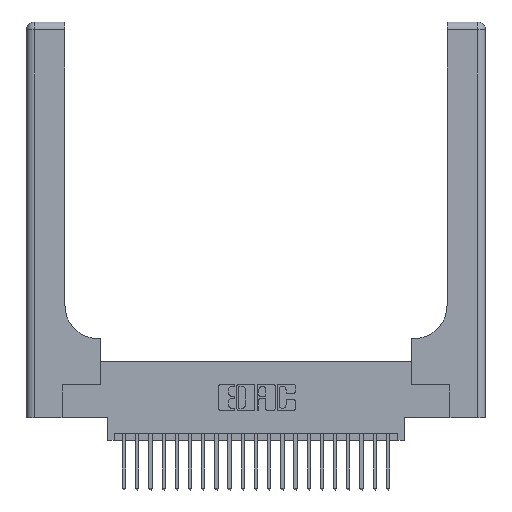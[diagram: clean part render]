
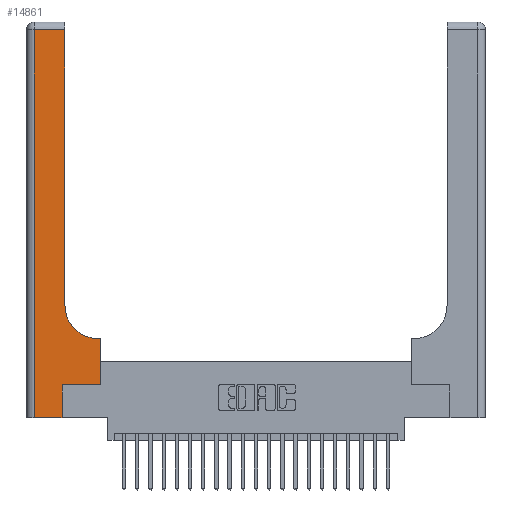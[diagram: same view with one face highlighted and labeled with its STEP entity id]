
A CAD part, top view. The second image highlights one B-rep face of the part: STEP entity #14861.
In plain terms, the highlighted planar face has unit normal (0, 0, 1).
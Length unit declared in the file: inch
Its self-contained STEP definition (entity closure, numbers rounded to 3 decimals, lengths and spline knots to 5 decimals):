
#70 = EDGE_LOOP ( 'NONE', ( #8513, #16734, #17218, #14912, #22025, #20427, #16551, #17496, #13132 ) ) ;
#830 = DIRECTION ( 'NONE',  ( -1., 0., 0. ) ) ;
#1219 = VECTOR ( 'NONE', #1689, 39.37008 ) ;
#1689 = DIRECTION ( 'NONE',  ( 1., 0., 0. ) ) ;
#1909 = VERTEX_POINT ( 'NONE', #11282 ) ;
#2113 = VERTEX_POINT ( 'NONE', #3494 ) ;
#2597 = VERTEX_POINT ( 'NONE', #21710 ) ;
#2657 = DIRECTION ( 'NONE',  ( 0., 0., -1. ) ) ;
#2665 = EDGE_CURVE ( 'NONE', #18563, #23103, #17933, .T. ) ;
#2709 = CARTESIAN_POINT ( 'NONE',  ( 0.5585, 0.25, 0.37 ) ) ;
#2771 = VECTOR ( 'NONE', #12998, 39.37008 ) ;
#3073 = FACE_OUTER_BOUND ( 'NONE', #70, .T. ) ;
#3276 = CIRCLE ( 'NONE', #20025, 0.25 ) ;
#3494 = CARTESIAN_POINT ( 'NONE',  ( 0.06, 2.94, 0.37 ) ) ;
#3606 = AXIS2_PLACEMENT_3D ( 'NONE', #9841, #6160, #8169 ) ;
#4570 = DIRECTION ( 'NONE',  ( 0., 1., 0. ) ) ;
#4891 = VECTOR ( 'NONE', #8653, 39.37008 ) ;
#5004 = EDGE_CURVE ( 'NONE', #17269, #2597, #8825, .T. ) ;
#5356 = VECTOR ( 'NONE', #14593, 39.37008 ) ;
#5906 = CARTESIAN_POINT ( 'NONE',  ( 0.06, 0., 0.37 ) ) ;
#6115 = EDGE_CURVE ( 'NONE', #1909, #17347, #9120, .T. ) ;
#6160 = DIRECTION ( 'NONE',  ( 0., 0., -1. ) ) ;
#6515 = LINE ( 'NONE', #20076, #21144 ) ;
#7162 = CARTESIAN_POINT ( 'NONE',  ( 0.2915, 3., 0.37 ) ) ;
#8169 = DIRECTION ( 'NONE',  ( -1., 0., 0. ) ) ;
#8288 = CARTESIAN_POINT ( 'NONE',  ( 0.5415, 0.85, 0.37 ) ) ;
#8387 = EDGE_CURVE ( 'NONE', #24023, #1909, #12891, .T. ) ;
#8513 = ORIENTED_EDGE ( 'NONE', *, *, #2665, .T. ) ;
#8653 = DIRECTION ( 'NONE',  ( 1., 0., 0. ) ) ;
#8825 = LINE ( 'NONE', #21282, #21071 ) ;
#9120 = LINE ( 'NONE', #22345, #4891 ) ;
#9154 = CARTESIAN_POINT ( 'NONE',  ( 0.269, 0., 0.37 ) ) ;
#9619 = EDGE_CURVE ( 'NONE', #2597, #18563, #3276, .T. ) ;
#9841 = CARTESIAN_POINT ( 'NONE',  ( 0., 3., 0.37 ) ) ;
#10125 = DIRECTION ( 'NONE',  ( 0., -1., 0. ) ) ;
#10188 = EDGE_CURVE ( 'NONE', #12968, #24023, #21439, .T. ) ;
#10872 = LINE ( 'NONE', #17648, #18021 ) ;
#10976 = CARTESIAN_POINT ( 'NONE',  ( 0.269, 0., 0.37 ) ) ;
#11282 = CARTESIAN_POINT ( 'NONE',  ( 0.269, 0.25, 0.37 ) ) ;
#11956 = LINE ( 'NONE', #2709, #17920 ) ;
#12891 = LINE ( 'NONE', #9154, #2771 ) ;
#12968 = VERTEX_POINT ( 'NONE', #5906 ) ;
#12998 = DIRECTION ( 'NONE',  ( 0., 1., 0. ) ) ;
#13132 = ORIENTED_EDGE ( 'NONE', *, *, #9619, .T. ) ;
#13579 = CARTESIAN_POINT ( 'NONE',  ( 0.5585, 0.25, 0.37 ) ) ;
#13702 = CARTESIAN_POINT ( 'NONE',  ( 0.2915, 0.85, 0.37 ) ) ;
#14593 = DIRECTION ( 'NONE',  ( 0., 1., 0. ) ) ;
#14861 = ADVANCED_FACE ( 'NONE', ( #3073 ), #21191, .F. ) ;
#14912 = ORIENTED_EDGE ( 'NONE', *, *, #10188, .T. ) ;
#15617 = EDGE_CURVE ( 'NONE', #17347, #17269, #11956, .T. ) ;
#16551 = ORIENTED_EDGE ( 'NONE', *, *, #15617, .T. ) ;
#16734 = ORIENTED_EDGE ( 'NONE', *, *, #17650, .T. ) ;
#17218 = ORIENTED_EDGE ( 'NONE', *, *, #23759, .T. ) ;
#17269 = VERTEX_POINT ( 'NONE', #20688 ) ;
#17347 = VERTEX_POINT ( 'NONE', #13579 ) ;
#17496 = ORIENTED_EDGE ( 'NONE', *, *, #5004, .T. ) ;
#17648 = CARTESIAN_POINT ( 'NONE',  ( 0.06, 3., 0.37 ) ) ;
#17650 = EDGE_CURVE ( 'NONE', #23103, #2113, #6515, .T. ) ;
#17920 = VECTOR ( 'NONE', #4570, 39.37008 ) ;
#17927 = DIRECTION ( 'NONE',  ( -1., 0., 0. ) ) ;
#17933 = LINE ( 'NONE', #7162, #5356 ) ;
#18021 = VECTOR ( 'NONE', #10125, 39.37008 ) ;
#18563 = VERTEX_POINT ( 'NONE', #13702 ) ;
#19824 = CARTESIAN_POINT ( 'NONE',  ( 0.2915, 2.94, 0.37 ) ) ;
#20025 = AXIS2_PLACEMENT_3D ( 'NONE', #8288, #2657, #23651 ) ;
#20076 = CARTESIAN_POINT ( 'NONE',  ( 0., 2.94, 0.37 ) ) ;
#20427 = ORIENTED_EDGE ( 'NONE', *, *, #6115, .T. ) ;
#20688 = CARTESIAN_POINT ( 'NONE',  ( 0.5585, 0.6, 0.37 ) ) ;
#20893 = CARTESIAN_POINT ( 'NONE',  ( 0., 0., 0.37 ) ) ;
#21071 = VECTOR ( 'NONE', #830, 39.37008 ) ;
#21144 = VECTOR ( 'NONE', #17927, 39.37008 ) ;
#21191 = PLANE ( 'NONE',  #3606 ) ;
#21282 = CARTESIAN_POINT ( 'NONE',  ( 0.2915, 0.6, 0.37 ) ) ;
#21439 = LINE ( 'NONE', #20893, #1219 ) ;
#21710 = CARTESIAN_POINT ( 'NONE',  ( 0.5415, 0.6, 0.37 ) ) ;
#22025 = ORIENTED_EDGE ( 'NONE', *, *, #8387, .T. ) ;
#22345 = CARTESIAN_POINT ( 'NONE',  ( 0.269, 0.25, 0.37 ) ) ;
#23103 = VERTEX_POINT ( 'NONE', #19824 ) ;
#23651 = DIRECTION ( 'NONE',  ( 1., 0., 0. ) ) ;
#23759 = EDGE_CURVE ( 'NONE', #2113, #12968, #10872, .T. ) ;
#24023 = VERTEX_POINT ( 'NONE', #10976 ) ;
